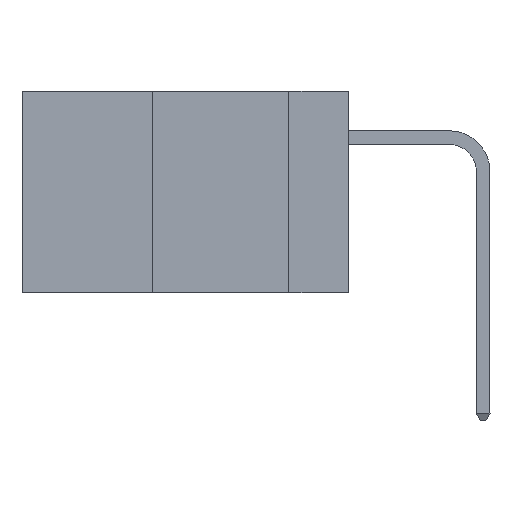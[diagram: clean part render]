
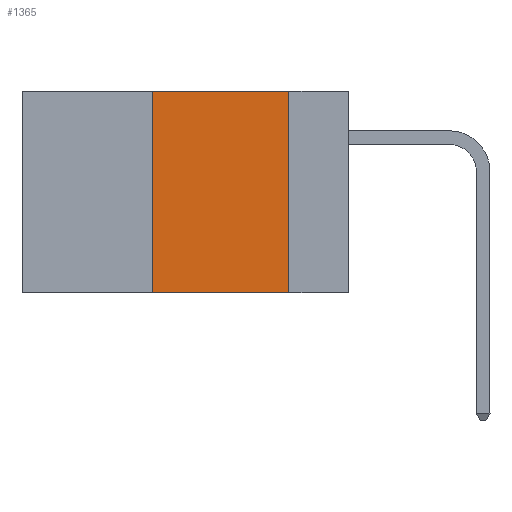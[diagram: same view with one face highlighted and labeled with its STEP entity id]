
A CAD part, left-side view. The second image highlights one B-rep face of the part: STEP entity #1365.
In plain terms, the highlighted planar face has unit normal (-1, 0, 0).
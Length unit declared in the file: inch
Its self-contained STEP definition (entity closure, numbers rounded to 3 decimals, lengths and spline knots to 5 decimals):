
#787 = VECTOR ( 'NONE', #12925, 39.37008 ) ;
#1234 = DIRECTION ( 'NONE',  ( 0., 0., -1. ) ) ;
#1365 = ADVANCED_FACE ( 'NONE', ( #18138 ), #10364, .F. ) ;
#2468 = CARTESIAN_POINT ( 'NONE',  ( 0., 0.6, 0. ) ) ;
#5098 = VECTOR ( 'NONE', #14375, 39.37008 ) ;
#5109 = ORIENTED_EDGE ( 'NONE', *, *, #7598, .T. ) ;
#6056 = ORIENTED_EDGE ( 'NONE', *, *, #7601, .F. ) ;
#7307 = CARTESIAN_POINT ( 'NONE',  ( 0., 0.11, -0.37 ) ) ;
#7598 = EDGE_CURVE ( 'NONE', #8571, #8616, #12836, .T. ) ;
#7601 = EDGE_CURVE ( 'NONE', #10226, #9424, #17682, .T. ) ;
#7662 = VECTOR ( 'NONE', #1234, 39.37008 ) ;
#8571 = VERTEX_POINT ( 'NONE', #18533 ) ;
#8616 = VERTEX_POINT ( 'NONE', #7307 ) ;
#8788 = DIRECTION ( 'NONE',  ( 0., 0., -1. ) ) ;
#9081 = ORIENTED_EDGE ( 'NONE', *, *, #13249, .F. ) ;
#9224 = CARTESIAN_POINT ( 'NONE',  ( 0., 0.11, 0. ) ) ;
#9424 = VERTEX_POINT ( 'NONE', #18482 ) ;
#9648 = EDGE_LOOP ( 'NONE', ( #9081, #6056, #17461, #5109 ) ) ;
#10118 = CARTESIAN_POINT ( 'NONE',  ( 0., 0.6, 0. ) ) ;
#10226 = VERTEX_POINT ( 'NONE', #10733 ) ;
#10364 = PLANE ( 'NONE',  #13305 ) ;
#10733 = CARTESIAN_POINT ( 'NONE',  ( 0., 0.36, 0. ) ) ;
#11272 = CARTESIAN_POINT ( 'NONE',  ( 0., 0.6, -0.37 ) ) ;
#12587 = LINE ( 'NONE', #18891, #13713 ) ;
#12836 = LINE ( 'NONE', #11272, #787 ) ;
#12925 = DIRECTION ( 'NONE',  ( 0., -1., 0. ) ) ;
#13249 = EDGE_CURVE ( 'NONE', #9424, #8616, #20327, .T. ) ;
#13305 = AXIS2_PLACEMENT_3D ( 'NONE', #2468, #16674, #8788 ) ;
#13713 = VECTOR ( 'NONE', #13726, 39.37008 ) ;
#13726 = DIRECTION ( 'NONE',  ( 0., 0., 1. ) ) ;
#14375 = DIRECTION ( 'NONE',  ( 0., -1., 0. ) ) ;
#16674 = DIRECTION ( 'NONE',  ( 1., 0., 0. ) ) ;
#16793 = EDGE_CURVE ( 'NONE', #8571, #10226, #12587, .T. ) ;
#17461 = ORIENTED_EDGE ( 'NONE', *, *, #16793, .F. ) ;
#17682 = LINE ( 'NONE', #10118, #5098 ) ;
#18138 = FACE_OUTER_BOUND ( 'NONE', #9648, .T. ) ;
#18482 = CARTESIAN_POINT ( 'NONE',  ( 0., 0.11, 0. ) ) ;
#18533 = CARTESIAN_POINT ( 'NONE',  ( 0., 0.36, -0.37 ) ) ;
#18891 = CARTESIAN_POINT ( 'NONE',  ( 0., 0.36, 0. ) ) ;
#20327 = LINE ( 'NONE', #9224, #7662 ) ;
